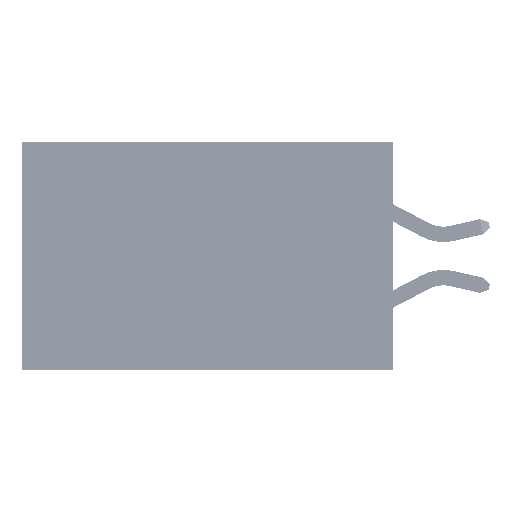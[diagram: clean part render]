
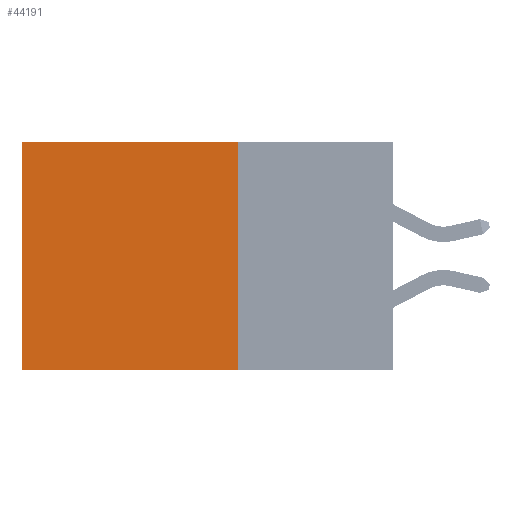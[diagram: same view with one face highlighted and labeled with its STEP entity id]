
A CAD part, left-side view. The second image highlights one B-rep face of the part: STEP entity #44191.
In plain terms, the highlighted planar face has unit normal (-1, 0, 0).
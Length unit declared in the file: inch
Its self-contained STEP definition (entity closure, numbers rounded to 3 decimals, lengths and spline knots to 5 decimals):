
#3429 = CARTESIAN_POINT ( 'NONE',  ( 0.2875, 0.6, -0.37 ) ) ;
#3487 = DIRECTION ( 'NONE',  ( 1., 0., 0. ) ) ;
#4833 = ORIENTED_EDGE ( 'NONE', *, *, #25409, .F. ) ;
#7427 = ORIENTED_EDGE ( 'NONE', *, *, #12154, .T. ) ;
#8257 = EDGE_LOOP ( 'NONE', ( #7427, #24676, #4833, #15890 ) ) ;
#9716 = CARTESIAN_POINT ( 'NONE',  ( 0.2875, 0.25, -0.37 ) ) ;
#11208 = CARTESIAN_POINT ( 'NONE',  ( 0.2875, 0.25, 0. ) ) ;
#12154 = EDGE_CURVE ( 'NONE', #24274, #39523, #15192, .T. ) ;
#15192 = LINE ( 'NONE', #15690, #27674 ) ;
#15554 = LINE ( 'NONE', #26767, #18492 ) ;
#15690 = CARTESIAN_POINT ( 'NONE',  ( 0.2875, 0.6, 0. ) ) ;
#15890 = ORIENTED_EDGE ( 'NONE', *, *, #38500, .T. ) ;
#17643 = VECTOR ( 'NONE', #34273, 39.37008 ) ;
#18492 = VECTOR ( 'NONE', #22293, 39.37008 ) ;
#18677 = FACE_OUTER_BOUND ( 'NONE', #8257, .T. ) ;
#19992 = LINE ( 'NONE', #35436, #17643 ) ;
#20169 = CARTESIAN_POINT ( 'NONE',  ( 0.2875, 0.25, -0.37 ) ) ;
#22293 = DIRECTION ( 'NONE',  ( 0., 0., -1. ) ) ;
#22415 = DIRECTION ( 'NONE',  ( 0., 0., -1. ) ) ;
#22669 = DIRECTION ( 'NONE',  ( 0., 0., -1. ) ) ;
#23904 = LINE ( 'NONE', #20169, #28669 ) ;
#24150 = DIRECTION ( 'NONE',  ( 0., 1., 0. ) ) ;
#24274 = VERTEX_POINT ( 'NONE', #40145 ) ;
#24676 = ORIENTED_EDGE ( 'NONE', *, *, #37639, .F. ) ;
#25409 = EDGE_CURVE ( 'NONE', #48356, #33508, #15554, .T. ) ;
#26767 = CARTESIAN_POINT ( 'NONE',  ( 0.2875, 0.25, 0. ) ) ;
#27674 = VECTOR ( 'NONE', #22415, 39.37008 ) ;
#28669 = VECTOR ( 'NONE', #24150, 39.37008 ) ;
#33508 = VERTEX_POINT ( 'NONE', #9716 ) ;
#34273 = DIRECTION ( 'NONE',  ( 0., 1., 0. ) ) ;
#35436 = CARTESIAN_POINT ( 'NONE',  ( 0.2875, 0.25, 0. ) ) ;
#37639 = EDGE_CURVE ( 'NONE', #33508, #39523, #23904, .T. ) ;
#38500 = EDGE_CURVE ( 'NONE', #48356, #24274, #19992, .T. ) ;
#39523 = VERTEX_POINT ( 'NONE', #3429 ) ;
#40145 = CARTESIAN_POINT ( 'NONE',  ( 0.2875, 0.6, 0. ) ) ;
#44191 = ADVANCED_FACE ( 'NONE', ( #18677 ), #45383, .F. ) ;
#45383 = PLANE ( 'NONE',  #45469 ) ;
#45469 = AXIS2_PLACEMENT_3D ( 'NONE', #45631, #3487, #22669 ) ;
#45631 = CARTESIAN_POINT ( 'NONE',  ( 0.2875, 0.25, 0. ) ) ;
#48356 = VERTEX_POINT ( 'NONE', #11208 ) ;
